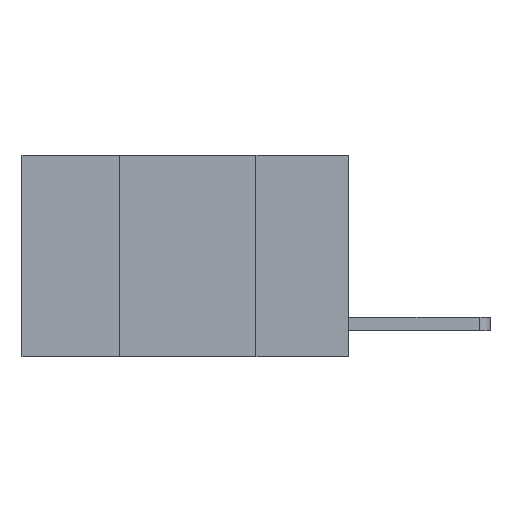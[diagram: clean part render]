
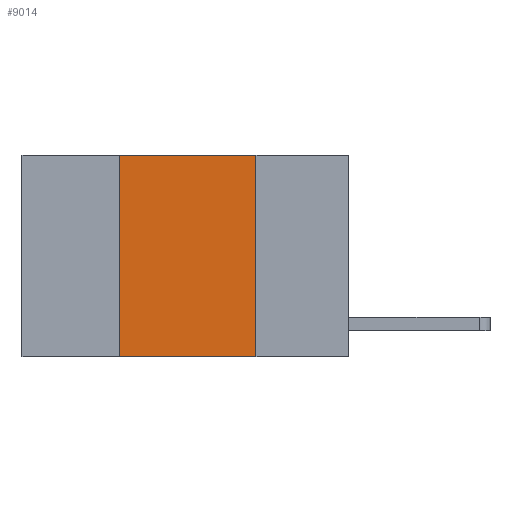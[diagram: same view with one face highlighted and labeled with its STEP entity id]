
A CAD part, left-side view. The second image highlights one B-rep face of the part: STEP entity #9014.
In plain terms, the highlighted planar face has unit normal (-1, 0, 0).
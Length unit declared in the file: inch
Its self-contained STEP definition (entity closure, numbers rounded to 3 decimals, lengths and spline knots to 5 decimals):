
#78 = LINE ( 'NONE', #5086, #5216 ) ;
#744 = DIRECTION ( 'NONE',  ( 0., 0., -1. ) ) ;
#1182 = VERTEX_POINT ( 'NONE', #7701 ) ;
#1209 = CARTESIAN_POINT ( 'NONE',  ( 0., 0.17, -0.37 ) ) ;
#1464 = CARTESIAN_POINT ( 'NONE',  ( 0., 0.6, 0. ) ) ;
#1630 = ORIENTED_EDGE ( 'NONE', *, *, #5959, .F. ) ;
#2857 = VERTEX_POINT ( 'NONE', #10889 ) ;
#2893 = CARTESIAN_POINT ( 'NONE',  ( 0., 0.42, 0. ) ) ;
#3136 = VECTOR ( 'NONE', #744, 39.37008 ) ;
#3215 = VECTOR ( 'NONE', #3763, 39.37008 ) ;
#3439 = CARTESIAN_POINT ( 'NONE',  ( 0., 0.17, 0. ) ) ;
#3762 = LINE ( 'NONE', #2893, #3215 ) ;
#3763 = DIRECTION ( 'NONE',  ( 0., 0., 1. ) ) ;
#4021 = DIRECTION ( 'NONE',  ( 0., -1., 0. ) ) ;
#4653 = VERTEX_POINT ( 'NONE', #1209 ) ;
#5028 = DIRECTION ( 'NONE',  ( 0., 0., -1. ) ) ;
#5086 = CARTESIAN_POINT ( 'NONE',  ( 0., 0.6, -0.37 ) ) ;
#5216 = VECTOR ( 'NONE', #10978, 39.37008 ) ;
#5552 = VECTOR ( 'NONE', #4021, 39.37008 ) ;
#5959 = EDGE_CURVE ( 'NONE', #2857, #8016, #7823, .T. ) ;
#6193 = EDGE_CURVE ( 'NONE', #8016, #4653, #10420, .T. ) ;
#6978 = AXIS2_PLACEMENT_3D ( 'NONE', #1464, #10072, #5028 ) ;
#7074 = FACE_OUTER_BOUND ( 'NONE', #11182, .T. ) ;
#7701 = CARTESIAN_POINT ( 'NONE',  ( 0., 0.42, -0.37 ) ) ;
#7789 = ORIENTED_EDGE ( 'NONE', *, *, #6193, .F. ) ;
#7823 = LINE ( 'NONE', #9067, #5552 ) ;
#7975 = ORIENTED_EDGE ( 'NONE', *, *, #9661, .T. ) ;
#8016 = VERTEX_POINT ( 'NONE', #3439 ) ;
#8398 = PLANE ( 'NONE',  #6978 ) ;
#8681 = EDGE_CURVE ( 'NONE', #1182, #2857, #3762, .T. ) ;
#9014 = ADVANCED_FACE ( 'NONE', ( #7074 ), #8398, .F. ) ;
#9067 = CARTESIAN_POINT ( 'NONE',  ( 0., 0.6, 0. ) ) ;
#9661 = EDGE_CURVE ( 'NONE', #1182, #4653, #78, .T. ) ;
#10072 = DIRECTION ( 'NONE',  ( 1., 0., 0. ) ) ;
#10420 = LINE ( 'NONE', #11089, #3136 ) ;
#10889 = CARTESIAN_POINT ( 'NONE',  ( 0., 0.42, 0. ) ) ;
#10978 = DIRECTION ( 'NONE',  ( 0., -1., 0. ) ) ;
#11089 = CARTESIAN_POINT ( 'NONE',  ( 0., 0.17, 0. ) ) ;
#11182 = EDGE_LOOP ( 'NONE', ( #7789, #1630, #11206, #7975 ) ) ;
#11206 = ORIENTED_EDGE ( 'NONE', *, *, #8681, .F. ) ;
